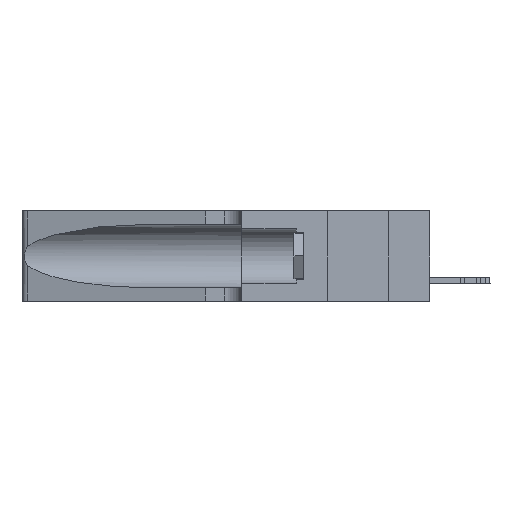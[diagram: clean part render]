
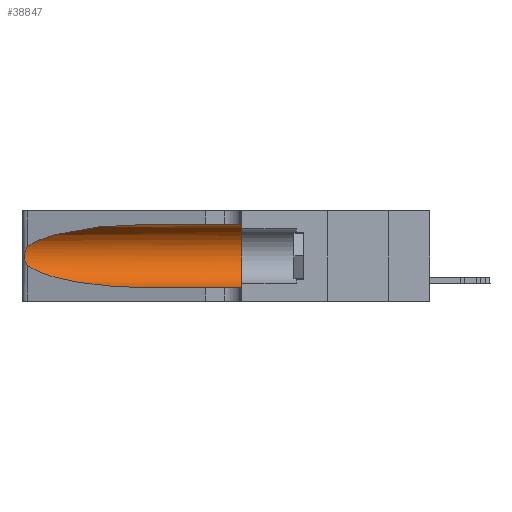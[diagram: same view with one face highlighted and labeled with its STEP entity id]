
A CAD part, left-side view. The second image highlights one B-rep face of the part: STEP entity #38847.
In plain terms, the highlighted cylindrical face has radius 3.308 mm (diameter 6.617 mm), a partial arc.
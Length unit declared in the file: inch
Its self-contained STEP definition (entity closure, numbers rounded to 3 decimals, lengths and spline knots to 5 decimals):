
#539 = VECTOR ( 'NONE', #33544, 39.37008 ) ;
#3338 = CARTESIAN_POINT ( 'NONE',  ( 0.1305, 1.61858, 0.31525 ) ) ;
#3379 = CARTESIAN_POINT ( 'NONE',  ( 0.26075, 1.23896, 0.19203 ) ) ;
#3875 = CARTESIAN_POINT ( 'NONE',  ( 0.26075, 1.23896, 0.178 ) ) ;
#4419 = ORIENTED_EDGE ( 'NONE', *, *, #37319, .T. ) ;
#4623 = CIRCLE ( 'NONE', #35734, 0.13025 ) ;
#4652 = VECTOR ( 'NONE', #18963, 39.37008 ) ;
#4718 = VERTEX_POINT ( 'NONE', #9887 ) ;
#9887 = CARTESIAN_POINT ( 'NONE',  ( 0.25487, 1.22718, 0.14631 ) ) ;
#10204 = ORIENTED_EDGE ( 'NONE', *, *, #41909, .F. ) ;
#10790 = EDGE_CURVE ( 'NONE', #40968, #38163, #34245, .T. ) ;
#11519 = VERTEX_POINT ( 'NONE', #12208 ) ;
#11637 = CARTESIAN_POINT ( 'NONE',  ( 0.18966, 0.96281, 0.05475 ) ) ;
#12208 = CARTESIAN_POINT ( 'NONE',  ( 0.25487, 1.22718, 0.22369 ) ) ;
#13821 = LINE ( 'NONE', #3338, #4652 ) ;
#14161 = ORIENTED_EDGE ( 'NONE', *, *, #48857, .T. ) ;
#15286 = CARTESIAN_POINT ( 'NONE',  ( 0.25555, 1.22994, 0.2215 ) ) ;
#15603 = CARTESIAN_POINT ( 'NONE',  ( 0.25487, 1.22718, 0.14631 ) ) ;
#15819 = VERTEX_POINT ( 'NONE', #36748 ) ;
#15994 =( BOUNDED_CURVE ( )  B_SPLINE_CURVE ( 3, ( #29840, #37622, #11637, #27264 ),
 .UNSPECIFIED., .F., .T. ) 
 B_SPLINE_CURVE_WITH_KNOTS ( ( 4, 4 ),
 ( 3.44316, 4.71239 ),
 .UNSPECIFIED. ) 
 CURVE ( )  GEOMETRIC_REPRESENTATION_ITEM ( )  RATIONAL_B_SPLINE_CURVE ( ( 1., 0.87, 0.87, 1. ) ) 
 REPRESENTATION_ITEM ( '' )  );
#16909 = CARTESIAN_POINT ( 'NONE',  ( 0.18966, 0.96281, 0.31525 ) ) ;
#18682 = CARTESIAN_POINT ( 'NONE',  ( 0.25856, 1.23593, 0.16098 ) ) ;
#18963 = DIRECTION ( 'NONE',  ( 0., -1., 0. ) ) ;
#20134 = CARTESIAN_POINT ( 'NONE',  ( 0.25487, 1.22718, 0.22369 ) ) ;
#22312 = CARTESIAN_POINT ( 'NONE',  ( 0.1305, 0.35, 0.185 ) ) ;
#22590 = CARTESIAN_POINT ( 'NONE',  ( 0.25789, 1.23486, 0.15765 ) ) ;
#23574 = VERTEX_POINT ( 'NONE', #23870 ) ;
#23870 = CARTESIAN_POINT ( 'NONE',  ( 0.1305, 0.72297, 0.31525 ) ) ;
#24976 = ORIENTED_EDGE ( 'NONE', *, *, #37428, .T. ) ;
#26558 = CARTESIAN_POINT ( 'NONE',  ( 0.25555, 1.22993, 0.14849 ) ) ;
#26726 = CARTESIAN_POINT ( 'NONE',  ( 0.25639, 1.23184, 0.21858 ) ) ;
#27203 = CARTESIAN_POINT ( 'NONE',  ( 0.26018, 1.23835, 0.19895 ) ) ;
#27264 = CARTESIAN_POINT ( 'NONE',  ( 0.1305, 0.72297, 0.05475 ) ) ;
#28557 = ORIENTED_EDGE ( 'NONE', *, *, #10790, .T. ) ;
#29124 = ORIENTED_EDGE ( 'NONE', *, *, #45774, .F. ) ;
#29561 = CARTESIAN_POINT ( 'NONE',  ( 0.1305, 1.61858, 0.185 ) ) ;
#29840 = CARTESIAN_POINT ( 'NONE',  ( 0.25487, 1.22718, 0.14631 ) ) ;
#30035 = DIRECTION ( 'NONE',  ( 0., 1., 0. ) ) ;
#30433 =( BOUNDED_CURVE ( )  B_SPLINE_CURVE ( 3, ( #37042, #16909, #47310, #20134 ),
 .UNSPECIFIED., .F., .F. ) 
 B_SPLINE_CURVE_WITH_KNOTS ( ( 4, 4 ),
 ( 1.5708, 2.84003 ),
 .UNSPECIFIED. ) 
 CURVE ( )  GEOMETRIC_REPRESENTATION_ITEM ( )  RATIONAL_B_SPLINE_CURVE ( ( 1., 0.87, 0.87, 1. ) ) 
 REPRESENTATION_ITEM ( '' )  );
#31705 = DIRECTION ( 'NONE',  ( 0., 0., -1. ) ) ;
#33135 = CARTESIAN_POINT ( 'NONE',  ( 0.1305, 0.35, 0.05475 ) ) ;
#33544 = DIRECTION ( 'NONE',  ( 0., -1., 0. ) ) ;
#33850 = DIRECTION ( 'NONE',  ( 0., -1., 0. ) ) ;
#34245 = LINE ( 'NONE', #45136, #539 ) ;
#34875 = CARTESIAN_POINT ( 'NONE',  ( 0.25787, 1.23484, 0.2124 ) ) ;
#35030 = CARTESIAN_POINT ( 'NONE',  ( 0.26017, 1.23833, 0.17102 ) ) ;
#35445 = CYLINDRICAL_SURFACE ( 'NONE', #45249, 0.13025 ) ;
#35734 = AXIS2_PLACEMENT_3D ( 'NONE', #22312, #30035, #45729 ) ;
#36748 = CARTESIAN_POINT ( 'NONE',  ( 0.1305, 0.35, 0.31525 ) ) ;
#37042 = CARTESIAN_POINT ( 'NONE',  ( 0.1305, 0.72297, 0.31525 ) ) ;
#37319 = EDGE_CURVE ( 'NONE', #4718, #40968, #15994, .T. ) ;
#37428 = EDGE_CURVE ( 'NONE', #23574, #11519, #30433, .T. ) ;
#37622 = CARTESIAN_POINT ( 'NONE',  ( 0.2373, 1.15595, 0.08982 ) ) ;
#38163 = VERTEX_POINT ( 'NONE', #33135 ) ;
#38847 = ADVANCED_FACE ( 'NONE', ( #40906 ), #35445, .F. ) ;
#40906 = FACE_OUTER_BOUND ( 'NONE', #46566, .T. ) ;
#40968 = VERTEX_POINT ( 'NONE', #48076 ) ;
#41909 = EDGE_CURVE ( 'NONE', #15819, #38163, #4623, .T. ) ;
#42708 = CARTESIAN_POINT ( 'NONE',  ( 0.25487, 1.22718, 0.22369 ) ) ;
#45136 = CARTESIAN_POINT ( 'NONE',  ( 0.1305, 1.61858, 0.05475 ) ) ;
#45249 = AXIS2_PLACEMENT_3D ( 'NONE', #29561, #33850, #31705 ) ;
#45729 = DIRECTION ( 'NONE',  ( 0., 0., 1. ) ) ;
#45774 = EDGE_CURVE ( 'NONE', #23574, #15819, #13821, .T. ) ;
#46022 = B_SPLINE_CURVE_WITH_KNOTS ( 'NONE', 3,
 ( #42708, #15286, #26726, #34875, #46672, #27203, #3379, #3875, #35030, #18682, #22590, #49902, #26558, #15603 ),
 .UNSPECIFIED., .F., .F.,
 ( 4, 2, 2, 2, 2, 2, 4 ),
 ( 0., 0.00027, 0.00053, 0.00107, 0.0016, 0.00187, 0.00214 ),
 .UNSPECIFIED. ) ;
#46566 = EDGE_LOOP ( 'NONE', ( #24976, #14161, #4419, #28557, #10204, #29124 ) ) ;
#46672 = CARTESIAN_POINT ( 'NONE',  ( 0.25854, 1.2359, 0.20912 ) ) ;
#47310 = CARTESIAN_POINT ( 'NONE',  ( 0.2373, 1.15595, 0.28018 ) ) ;
#48076 = CARTESIAN_POINT ( 'NONE',  ( 0.1305, 0.72297, 0.05475 ) ) ;
#48857 = EDGE_CURVE ( 'NONE', #11519, #4718, #46022, .T. ) ;
#49902 = CARTESIAN_POINT ( 'NONE',  ( 0.25639, 1.23186, 0.15144 ) ) ;
